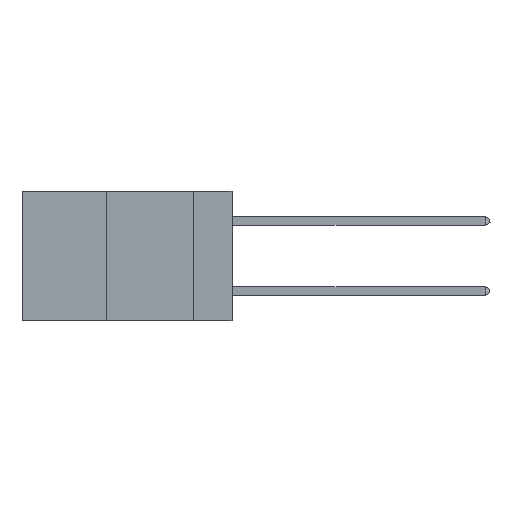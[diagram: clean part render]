
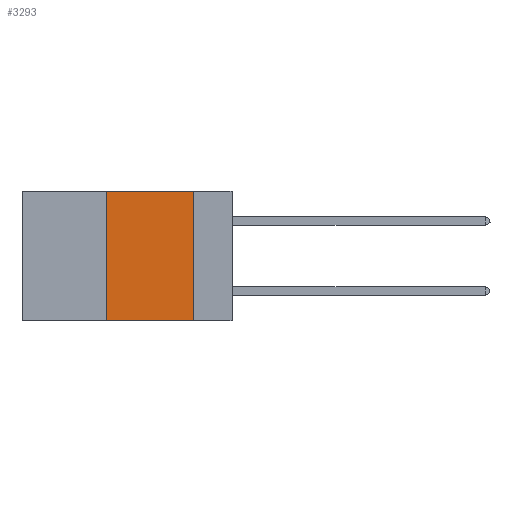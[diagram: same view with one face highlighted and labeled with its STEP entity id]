
A CAD part, left-side view. The second image highlights one B-rep face of the part: STEP entity #3293.
In plain terms, the highlighted planar face has unit normal (-1, 0, 0).
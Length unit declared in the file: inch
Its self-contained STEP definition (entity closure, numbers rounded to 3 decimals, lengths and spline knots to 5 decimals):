
#711 = DIRECTION ( 'NONE',  ( 0., -1., 0. ) ) ;
#840 = DIRECTION ( 'NONE',  ( 0., 0., -1. ) ) ;
#1038 = DIRECTION ( 'NONE',  ( 1., 0., 0. ) ) ;
#1358 = CARTESIAN_POINT ( 'NONE',  ( 0., 0.6, 0. ) ) ;
#3286 = PLANE ( 'NONE',  #5805 ) ;
#3293 = ADVANCED_FACE ( 'NONE', ( #14746 ), #3286, .F. ) ;
#3943 = ORIENTED_EDGE ( 'NONE', *, *, #22723, .F. ) ;
#4527 = ORIENTED_EDGE ( 'NONE', *, *, #18902, .F. ) ;
#4647 = VERTEX_POINT ( 'NONE', #20326 ) ;
#4719 = VERTEX_POINT ( 'NONE', #7300 ) ;
#4814 = EDGE_CURVE ( 'NONE', #4647, #8891, #16266, .T. ) ;
#5092 = VERTEX_POINT ( 'NONE', #12903 ) ;
#5372 = VECTOR ( 'NONE', #8251, 39.37008 ) ;
#5805 = AXIS2_PLACEMENT_3D ( 'NONE', #1358, #1038, #840 ) ;
#6291 = CARTESIAN_POINT ( 'NONE',  ( 0., 0.36, 0. ) ) ;
#7057 = DIRECTION ( 'NONE',  ( 0., 0., -1. ) ) ;
#7300 = CARTESIAN_POINT ( 'NONE',  ( 0., 0.36, -0.37 ) ) ;
#8251 = DIRECTION ( 'NONE',  ( 0., 0., 1. ) ) ;
#8608 = CARTESIAN_POINT ( 'NONE',  ( 0., 0.11, 0. ) ) ;
#8891 = VERTEX_POINT ( 'NONE', #14032 ) ;
#9336 = VECTOR ( 'NONE', #711, 39.37008 ) ;
#10296 = ORIENTED_EDGE ( 'NONE', *, *, #14149, .T. ) ;
#10326 = CARTESIAN_POINT ( 'NONE',  ( 0., 0.6, -0.37 ) ) ;
#11245 = LINE ( 'NONE', #11528, #20581 ) ;
#11528 = CARTESIAN_POINT ( 'NONE',  ( 0., 0.6, 0. ) ) ;
#12903 = CARTESIAN_POINT ( 'NONE',  ( 0., 0.36, 0. ) ) ;
#13389 = DIRECTION ( 'NONE',  ( 0., -1., 0. ) ) ;
#14032 = CARTESIAN_POINT ( 'NONE',  ( 0., 0.11, -0.37 ) ) ;
#14149 = EDGE_CURVE ( 'NONE', #4719, #8891, #19901, .T. ) ;
#14746 = FACE_OUTER_BOUND ( 'NONE', #23658, .T. ) ;
#14923 = LINE ( 'NONE', #6291, #5372 ) ;
#16266 = LINE ( 'NONE', #8608, #20610 ) ;
#18902 = EDGE_CURVE ( 'NONE', #5092, #4647, #11245, .T. ) ;
#19901 = LINE ( 'NONE', #10326, #9336 ) ;
#20326 = CARTESIAN_POINT ( 'NONE',  ( 0., 0.11, 0. ) ) ;
#20581 = VECTOR ( 'NONE', #13389, 39.37008 ) ;
#20610 = VECTOR ( 'NONE', #7057, 39.37008 ) ;
#22723 = EDGE_CURVE ( 'NONE', #4719, #5092, #14923, .T. ) ;
#23396 = ORIENTED_EDGE ( 'NONE', *, *, #4814, .F. ) ;
#23658 = EDGE_LOOP ( 'NONE', ( #23396, #4527, #3943, #10296 ) ) ;
